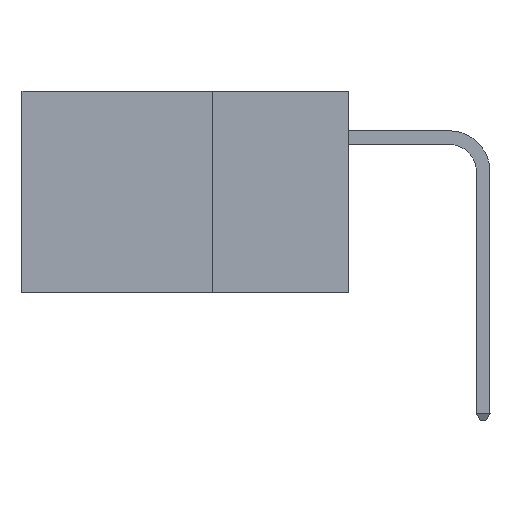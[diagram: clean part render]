
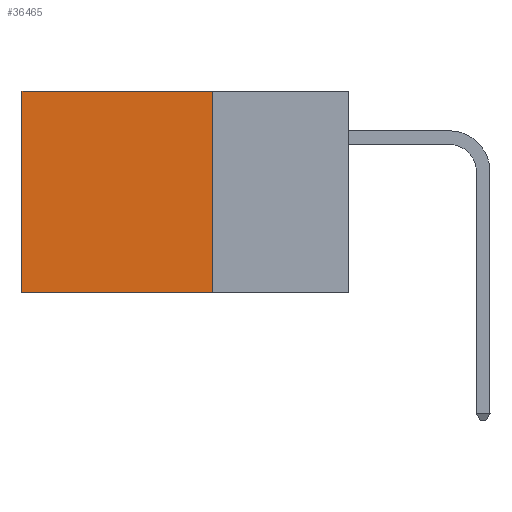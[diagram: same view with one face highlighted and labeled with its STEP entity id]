
A CAD part, left-side view. The second image highlights one B-rep face of the part: STEP entity #36465.
In plain terms, the highlighted planar face has unit normal (-1, 0, 0).
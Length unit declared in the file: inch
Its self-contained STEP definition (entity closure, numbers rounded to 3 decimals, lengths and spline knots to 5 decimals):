
#1051 = VERTEX_POINT ( 'NONE', #4225 ) ;
#3047 = LINE ( 'NONE', #45807, #36860 ) ;
#3827 = CARTESIAN_POINT ( 'NONE',  ( 0.2875, 0.25, 0. ) ) ;
#4225 = CARTESIAN_POINT ( 'NONE',  ( 0.2875, 0.25, 0. ) ) ;
#5955 = VECTOR ( 'NONE', #7043, 39.37008 ) ;
#7043 = DIRECTION ( 'NONE',  ( 0., 0., -1. ) ) ;
#11529 = DIRECTION ( 'NONE',  ( 0., 1., 0. ) ) ;
#11838 = EDGE_CURVE ( 'NONE', #13994, #15764, #14539, .T. ) ;
#13994 = VERTEX_POINT ( 'NONE', #15741 ) ;
#14539 = LINE ( 'NONE', #21788, #5955 ) ;
#14973 = CARTESIAN_POINT ( 'NONE',  ( 0.2875, 0.25, 0. ) ) ;
#15561 = FACE_OUTER_BOUND ( 'NONE', #26852, .T. ) ;
#15741 = CARTESIAN_POINT ( 'NONE',  ( 0.2875, 0.6, 0. ) ) ;
#15764 = VERTEX_POINT ( 'NONE', #45732 ) ;
#16997 = ORIENTED_EDGE ( 'NONE', *, *, #18938, .F. ) ;
#18125 = EDGE_CURVE ( 'NONE', #1051, #32589, #40986, .T. ) ;
#18415 = LINE ( 'NONE', #42187, #44222 ) ;
#18938 = EDGE_CURVE ( 'NONE', #32589, #15764, #3047, .T. ) ;
#20038 = VECTOR ( 'NONE', #25989, 39.37008 ) ;
#21054 = EDGE_CURVE ( 'NONE', #1051, #13994, #18415, .T. ) ;
#21076 = AXIS2_PLACEMENT_3D ( 'NONE', #3827, #46100, #26592 ) ;
#21701 = ORIENTED_EDGE ( 'NONE', *, *, #18125, .F. ) ;
#21788 = CARTESIAN_POINT ( 'NONE',  ( 0.2875, 0.6, 0. ) ) ;
#25989 = DIRECTION ( 'NONE',  ( 0., 0., -1. ) ) ;
#26592 = DIRECTION ( 'NONE',  ( 0., 0., -1. ) ) ;
#26852 = EDGE_LOOP ( 'NONE', ( #47102, #16997, #21701, #45758 ) ) ;
#32589 = VERTEX_POINT ( 'NONE', #42693 ) ;
#33434 = DIRECTION ( 'NONE',  ( 0., 1., 0. ) ) ;
#34077 = PLANE ( 'NONE',  #21076 ) ;
#36465 = ADVANCED_FACE ( 'NONE', ( #15561 ), #34077, .F. ) ;
#36860 = VECTOR ( 'NONE', #11529, 39.37008 ) ;
#40986 = LINE ( 'NONE', #14973, #20038 ) ;
#42187 = CARTESIAN_POINT ( 'NONE',  ( 0.2875, 0.25, 0. ) ) ;
#42693 = CARTESIAN_POINT ( 'NONE',  ( 0.2875, 0.25, -0.37 ) ) ;
#44222 = VECTOR ( 'NONE', #33434, 39.37008 ) ;
#45732 = CARTESIAN_POINT ( 'NONE',  ( 0.2875, 0.6, -0.37 ) ) ;
#45758 = ORIENTED_EDGE ( 'NONE', *, *, #21054, .T. ) ;
#45807 = CARTESIAN_POINT ( 'NONE',  ( 0.2875, 0.25, -0.37 ) ) ;
#46100 = DIRECTION ( 'NONE',  ( 1., 0., 0. ) ) ;
#47102 = ORIENTED_EDGE ( 'NONE', *, *, #11838, .T. ) ;
